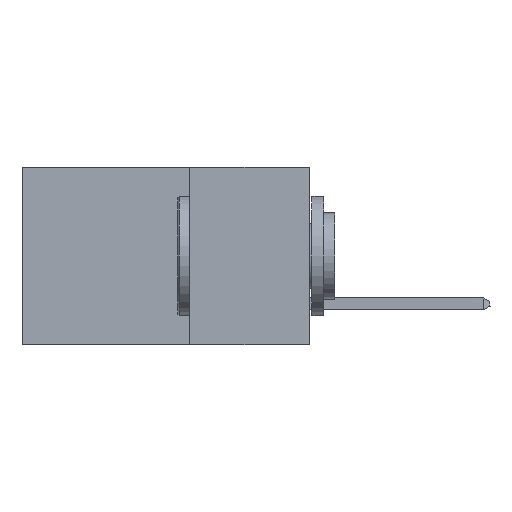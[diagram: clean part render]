
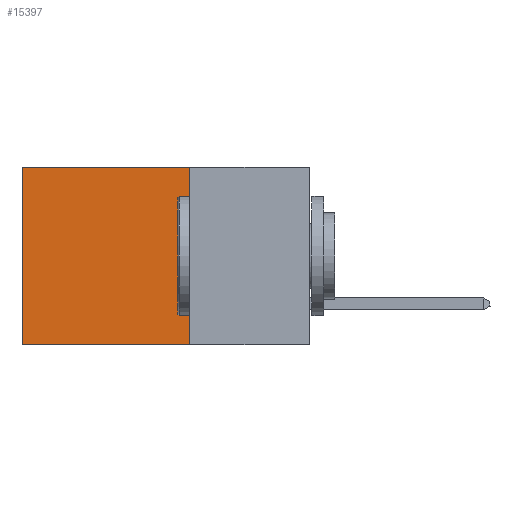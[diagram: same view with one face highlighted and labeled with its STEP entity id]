
A CAD part, left-side view. The second image highlights one B-rep face of the part: STEP entity #15397.
In plain terms, the highlighted planar face has unit normal (-1, 0, 0).
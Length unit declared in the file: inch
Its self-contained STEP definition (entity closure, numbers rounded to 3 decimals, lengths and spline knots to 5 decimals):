
#1405 = FACE_OUTER_BOUND ( 'NONE', #13061, .T. ) ;
#1708 = AXIS2_PLACEMENT_3D ( 'NONE', #4830, #10102, #20642 ) ;
#2021 = VERTEX_POINT ( 'NONE', #9258 ) ;
#2445 = CARTESIAN_POINT ( 'NONE',  ( 0.2875, 0.25, 0. ) ) ;
#2571 = CARTESIAN_POINT ( 'NONE',  ( 0.2875, 0.6, -0.37 ) ) ;
#3127 = DIRECTION ( 'NONE',  ( 0., 0., -1. ) ) ;
#3135 = VERTEX_POINT ( 'NONE', #2571 ) ;
#3670 = VECTOR ( 'NONE', #3127, 39.37008 ) ;
#3749 = EDGE_CURVE ( 'NONE', #9712, #3135, #20175, .T. ) ;
#4830 = CARTESIAN_POINT ( 'NONE',  ( 0.2875, 0.25, 0. ) ) ;
#5360 = DIRECTION ( 'NONE',  ( 0., 1., 0. ) ) ;
#5561 = ORIENTED_EDGE ( 'NONE', *, *, #9726, .T. ) ;
#5579 = EDGE_CURVE ( 'NONE', #2021, #9712, #8177, .T. ) ;
#5730 = ORIENTED_EDGE ( 'NONE', *, *, #7478, .T. ) ;
#6489 = CARTESIAN_POINT ( 'NONE',  ( 0.2875, 0.25, 0. ) ) ;
#6552 = CARTESIAN_POINT ( 'NONE',  ( 0.2875, 0.6, 0. ) ) ;
#6628 = ORIENTED_EDGE ( 'NONE', *, *, #5579, .F. ) ;
#7478 = EDGE_CURVE ( 'NONE', #14022, #3135, #21994, .T. ) ;
#8177 = LINE ( 'NONE', #2445, #15393 ) ;
#9258 = CARTESIAN_POINT ( 'NONE',  ( 0.2875, 0.25, 0. ) ) ;
#9712 = VERTEX_POINT ( 'NONE', #13629 ) ;
#9726 = EDGE_CURVE ( 'NONE', #2021, #14022, #20224, .T. ) ;
#9858 = PLANE ( 'NONE',  #1708 ) ;
#10102 = DIRECTION ( 'NONE',  ( 1., 0., 0. ) ) ;
#12996 = DIRECTION ( 'NONE',  ( 0., 0., -1. ) ) ;
#13061 = EDGE_LOOP ( 'NONE', ( #5730, #18646, #6628, #5561 ) ) ;
#13629 = CARTESIAN_POINT ( 'NONE',  ( 0.2875, 0.25, -0.37 ) ) ;
#13862 = VECTOR ( 'NONE', #17181, 39.37008 ) ;
#14022 = VERTEX_POINT ( 'NONE', #20127 ) ;
#15393 = VECTOR ( 'NONE', #12996, 39.37008 ) ;
#15397 = ADVANCED_FACE ( 'NONE', ( #1405 ), #9858, .F. ) ;
#17181 = DIRECTION ( 'NONE',  ( 0., 1., 0. ) ) ;
#18646 = ORIENTED_EDGE ( 'NONE', *, *, #3749, .F. ) ;
#18869 = CARTESIAN_POINT ( 'NONE',  ( 0.2875, 0.25, -0.37 ) ) ;
#19602 = VECTOR ( 'NONE', #5360, 39.37008 ) ;
#20127 = CARTESIAN_POINT ( 'NONE',  ( 0.2875, 0.6, 0. ) ) ;
#20175 = LINE ( 'NONE', #18869, #19602 ) ;
#20224 = LINE ( 'NONE', #6489, #13862 ) ;
#20642 = DIRECTION ( 'NONE',  ( 0., 0., -1. ) ) ;
#21994 = LINE ( 'NONE', #6552, #3670 ) ;
